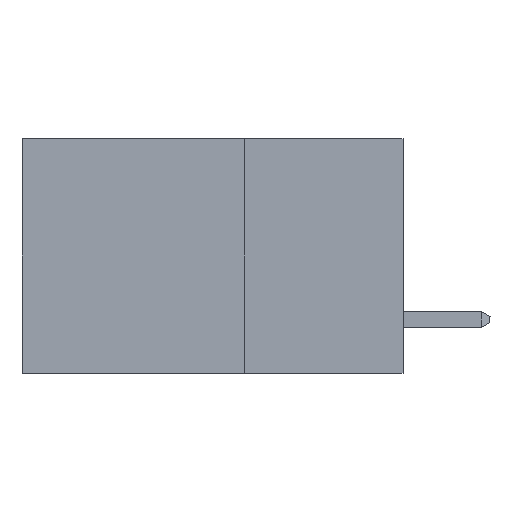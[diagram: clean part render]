
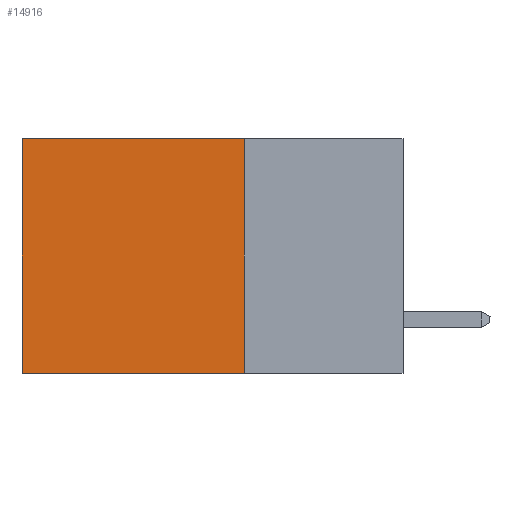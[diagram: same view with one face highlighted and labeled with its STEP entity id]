
A CAD part, left-side view. The second image highlights one B-rep face of the part: STEP entity #14916.
In plain terms, the highlighted planar face has unit normal (-1, 0, 0).
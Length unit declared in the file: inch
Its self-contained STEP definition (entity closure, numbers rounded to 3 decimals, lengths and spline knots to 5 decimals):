
#161 = EDGE_CURVE ( 'NONE', #30608, #6202, #26840, .T. ) ;
#946 = VECTOR ( 'NONE', #16431, 39.37008 ) ;
#1907 = VERTEX_POINT ( 'NONE', #15971 ) ;
#1964 = LINE ( 'NONE', #7664, #13791 ) ;
#4375 = AXIS2_PLACEMENT_3D ( 'NONE', #6463, #13275, #11071 ) ;
#4594 = CARTESIAN_POINT ( 'NONE',  ( 0.2875, 0.25, 0. ) ) ;
#6202 = VERTEX_POINT ( 'NONE', #25598 ) ;
#6463 = CARTESIAN_POINT ( 'NONE',  ( 0.2875, 0.25, 0. ) ) ;
#7664 = CARTESIAN_POINT ( 'NONE',  ( 0.2875, 0.6, 0. ) ) ;
#7682 = FACE_OUTER_BOUND ( 'NONE', #17674, .T. ) ;
#8074 = VECTOR ( 'NONE', #19302, 39.37008 ) ;
#9921 = CARTESIAN_POINT ( 'NONE',  ( 0.2875, 0.25, 0. ) ) ;
#10333 = ORIENTED_EDGE ( 'NONE', *, *, #161, .F. ) ;
#11071 = DIRECTION ( 'NONE',  ( 0., 0., -1. ) ) ;
#11235 = DIRECTION ( 'NONE',  ( 0., 1., 0. ) ) ;
#12116 = EDGE_CURVE ( 'NONE', #12151, #1907, #26222, .T. ) ;
#12151 = VERTEX_POINT ( 'NONE', #17013 ) ;
#13275 = DIRECTION ( 'NONE',  ( 1., 0., 0. ) ) ;
#13791 = VECTOR ( 'NONE', #27464, 39.37008 ) ;
#13817 = ORIENTED_EDGE ( 'NONE', *, *, #31068, .T. ) ;
#14916 = ADVANCED_FACE ( 'NONE', ( #7682 ), #30851, .F. ) ;
#15971 = CARTESIAN_POINT ( 'NONE',  ( 0.2875, 0.6, 0. ) ) ;
#15989 = ORIENTED_EDGE ( 'NONE', *, *, #30999, .F. ) ;
#16431 = DIRECTION ( 'NONE',  ( 0., 1., 0. ) ) ;
#17013 = CARTESIAN_POINT ( 'NONE',  ( 0.2875, 0.25, 0. ) ) ;
#17674 = EDGE_LOOP ( 'NONE', ( #13817, #10333, #15989, #17962 ) ) ;
#17962 = ORIENTED_EDGE ( 'NONE', *, *, #12116, .T. ) ;
#17977 = VECTOR ( 'NONE', #11235, 39.37008 ) ;
#18754 = LINE ( 'NONE', #9921, #8074 ) ;
#19302 = DIRECTION ( 'NONE',  ( 0., 0., -1. ) ) ;
#21785 = CARTESIAN_POINT ( 'NONE',  ( 0.2875, 0.25, -0.37 ) ) ;
#25598 = CARTESIAN_POINT ( 'NONE',  ( 0.2875, 0.6, -0.37 ) ) ;
#26222 = LINE ( 'NONE', #4594, #946 ) ;
#26840 = LINE ( 'NONE', #21785, #17977 ) ;
#27464 = DIRECTION ( 'NONE',  ( 0., 0., -1. ) ) ;
#29761 = CARTESIAN_POINT ( 'NONE',  ( 0.2875, 0.25, -0.37 ) ) ;
#30608 = VERTEX_POINT ( 'NONE', #29761 ) ;
#30851 = PLANE ( 'NONE',  #4375 ) ;
#30999 = EDGE_CURVE ( 'NONE', #12151, #30608, #18754, .T. ) ;
#31068 = EDGE_CURVE ( 'NONE', #1907, #6202, #1964, .T. ) ;
